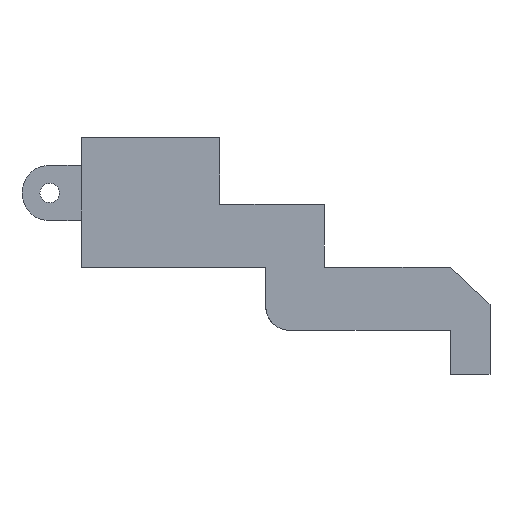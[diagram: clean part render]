
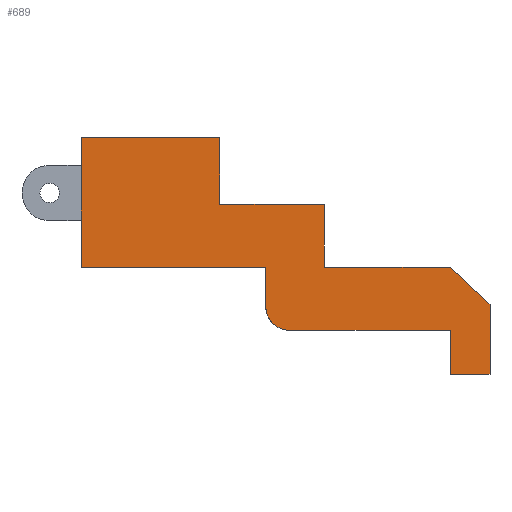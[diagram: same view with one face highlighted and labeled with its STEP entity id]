
A CAD part, front view. The second image highlights one B-rep face of the part: STEP entity #689.
In plain terms, the highlighted planar face has unit normal (0, -1, 0).
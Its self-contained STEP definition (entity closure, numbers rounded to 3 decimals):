
#36=CIRCLE('',#740,1.9);
#72=FACE_OUTER_BOUND('',#112,.T.);
#112=EDGE_LOOP('',(#611,#612,#613,#614,#615,#616,#617,#618,#619,#620,#621,
#622,#623,#624));
#118=LINE('',#946,#200);
#121=LINE('',#951,#203);
#125=LINE('',#959,#207);
#128=LINE('',#965,#210);
#168=LINE('',#1068,#250);
#176=LINE('',#1089,#258);
#177=LINE('',#1092,#259);
#180=LINE('',#1098,#262);
#184=LINE('',#1105,#266);
#186=LINE('',#1108,#268);
#187=LINE('',#1111,#269);
#190=LINE('',#1117,#272);
#193=LINE('',#1122,#275);
#200=VECTOR('',#763,10.);
#203=VECTOR('',#768,10.);
#207=VECTOR('',#774,10.);
#210=VECTOR('',#779,10.);
#250=VECTOR('',#873,10.);
#258=VECTOR('',#895,10.);
#259=VECTOR('',#898,10.);
#262=VECTOR('',#903,10.);
#266=VECTOR('',#909,10.);
#268=VECTOR('',#913,10.);
#269=VECTOR('',#916,10.);
#272=VECTOR('',#921,10.);
#275=VECTOR('',#926,10.);
#281=VERTEX_POINT('',#943);
#282=VERTEX_POINT('',#945);
#283=VERTEX_POINT('',#949);
#286=VERTEX_POINT('',#957);
#288=VERTEX_POINT('',#963);
#323=VERTEX_POINT('',#1065);
#324=VERTEX_POINT('',#1067);
#328=VERTEX_POINT('',#1081);
#329=VERTEX_POINT('',#1083);
#331=VERTEX_POINT('',#1091);
#333=VERTEX_POINT('',#1097);
#335=VERTEX_POINT('',#1103);
#336=VERTEX_POINT('',#1110);
#338=VERTEX_POINT('',#1116);
#345=EDGE_CURVE('',#282,#281,#118,.T.);
#348=EDGE_CURVE('',#283,#281,#121,.T.);
#352=EDGE_CURVE('',#286,#283,#125,.T.);
#355=EDGE_CURVE('',#288,#286,#128,.T.);
#405=EDGE_CURVE('',#323,#324,#168,.T.);
#413=EDGE_CURVE('',#328,#329,#36,.T.);
#416=EDGE_CURVE('',#282,#328,#176,.T.);
#417=EDGE_CURVE('',#331,#288,#177,.T.);
#420=EDGE_CURVE('',#333,#331,#180,.T.);
#424=EDGE_CURVE('',#335,#333,#184,.T.);
#426=EDGE_CURVE('',#324,#335,#186,.T.);
#427=EDGE_CURVE('',#336,#323,#187,.T.);
#430=EDGE_CURVE('',#338,#336,#190,.T.);
#433=EDGE_CURVE('',#329,#338,#193,.T.);
#611=ORIENTED_EDGE('',*,*,#413,.F.);
#612=ORIENTED_EDGE('',*,*,#416,.F.);
#613=ORIENTED_EDGE('',*,*,#345,.T.);
#614=ORIENTED_EDGE('',*,*,#348,.F.);
#615=ORIENTED_EDGE('',*,*,#352,.F.);
#616=ORIENTED_EDGE('',*,*,#355,.F.);
#617=ORIENTED_EDGE('',*,*,#417,.F.);
#618=ORIENTED_EDGE('',*,*,#420,.F.);
#619=ORIENTED_EDGE('',*,*,#424,.F.);
#620=ORIENTED_EDGE('',*,*,#426,.F.);
#621=ORIENTED_EDGE('',*,*,#405,.F.);
#622=ORIENTED_EDGE('',*,*,#427,.F.);
#623=ORIENTED_EDGE('',*,*,#430,.F.);
#624=ORIENTED_EDGE('',*,*,#433,.F.);
#654=PLANE('',#751);
#689=ADVANCED_FACE('',(#72),#654,.F.);
#740=AXIS2_PLACEMENT_3D('',#1084,#888,#889);
#751=AXIS2_PLACEMENT_3D('',#1125,#930,#931);
#763=DIRECTION('',(0.,0.,-1.));
#768=DIRECTION('',(-1.,0.,0.));
#774=DIRECTION('',(0.,0.,-1.));
#779=DIRECTION('',(0.731,0.,-0.682));
#873=DIRECTION('',(1.,0.,0.));
#888=DIRECTION('center_axis',(0.,1.,0.));
#889=DIRECTION('ref_axis',(0.,0.,-1.));
#895=DIRECTION('',(-1.,0.,0.));
#898=DIRECTION('',(1.,0.,0.));
#903=DIRECTION('',(0.,0.,-1.));
#909=DIRECTION('',(1.,0.,0.));
#913=DIRECTION('',(0.,0.,-1.));
#916=DIRECTION('',(0.,0.,1.));
#921=DIRECTION('',(-1.,0.,0.));
#926=DIRECTION('',(0.,0.,1.));
#930=DIRECTION('center_axis',(0.,1.,0.));
#931=DIRECTION('ref_axis',(1.,0.,0.));
#943=CARTESIAN_POINT('',(14.65,0.,-11.15));
#945=CARTESIAN_POINT('',(14.65,0.,-7.65));
#946=CARTESIAN_POINT('',(14.65,0.,-7.65));
#949=CARTESIAN_POINT('',(17.795,0.,-11.15));
#951=CARTESIAN_POINT('',(17.795,0.,-11.15));
#957=CARTESIAN_POINT('',(17.795,0.,-5.583));
#959=CARTESIAN_POINT('',(17.795,0.,-5.583));
#963=CARTESIAN_POINT('',(14.65,0.,-2.65));
#965=CARTESIAN_POINT('',(14.65,0.,-2.65));
#1065=CARTESIAN_POINT('',(-14.65,0.,7.65));
#1067=CARTESIAN_POINT('',(-3.65,0.,7.65));
#1068=CARTESIAN_POINT('',(-14.65,0.,7.65));
#1081=CARTESIAN_POINT('',(1.9,0.,-7.65));
#1083=CARTESIAN_POINT('',(0.,0.,-5.75));
#1084=CARTESIAN_POINT('Origin',(1.9,0.,-5.75));
#1089=CARTESIAN_POINT('',(14.65,0.,-7.65));
#1091=CARTESIAN_POINT('',(4.65,0.,-2.65));
#1092=CARTESIAN_POINT('',(4.65,0.,-2.65));
#1097=CARTESIAN_POINT('',(4.65,0.,2.35));
#1098=CARTESIAN_POINT('',(4.65,0.,2.35));
#1103=CARTESIAN_POINT('',(-3.65,0.,2.35));
#1105=CARTESIAN_POINT('',(-3.65,0.,2.35));
#1108=CARTESIAN_POINT('',(-3.65,0.,7.65));
#1110=CARTESIAN_POINT('',(-14.65,0.,-2.65));
#1111=CARTESIAN_POINT('',(-14.65,0.,-2.65));
#1116=CARTESIAN_POINT('',(0.,0.,-2.65));
#1117=CARTESIAN_POINT('',(0.,0.,-2.65));
#1122=CARTESIAN_POINT('',(0.,0.,-5.75));
#1125=CARTESIAN_POINT('Origin',(0.,0.,0.));
